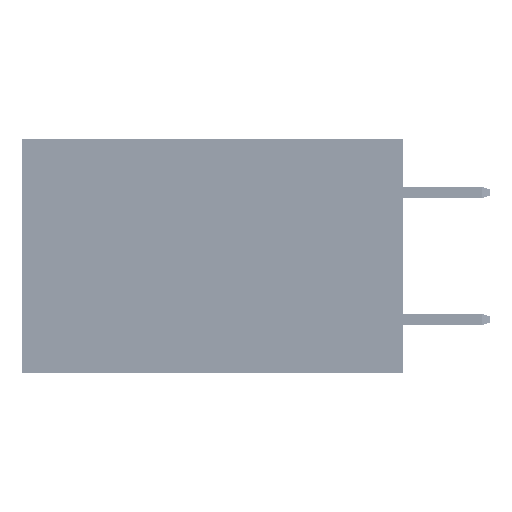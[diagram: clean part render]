
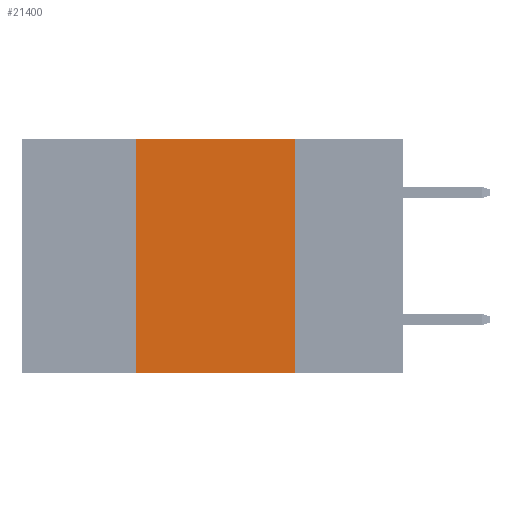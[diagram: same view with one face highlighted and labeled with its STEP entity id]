
A CAD part, left-side view. The second image highlights one B-rep face of the part: STEP entity #21400.
In plain terms, the highlighted planar face has unit normal (-1, 0, 0).
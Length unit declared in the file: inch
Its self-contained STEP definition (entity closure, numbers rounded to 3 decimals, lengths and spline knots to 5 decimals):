
#2221 = VERTEX_POINT ( 'NONE', #44517 ) ;
#2843 = CARTESIAN_POINT ( 'NONE',  ( 0., 0.17, 0. ) ) ;
#5233 = ORIENTED_EDGE ( 'NONE', *, *, #7562, .F. ) ;
#5838 = CARTESIAN_POINT ( 'NONE',  ( 0., 0.6, 0. ) ) ;
#6639 = CARTESIAN_POINT ( 'NONE',  ( 0., 0.6, -0.37 ) ) ;
#7511 = DIRECTION ( 'NONE',  ( 1., 0., 0. ) ) ;
#7562 = EDGE_CURVE ( 'NONE', #13985, #13422, #18154, .T. ) ;
#7747 = DIRECTION ( 'NONE',  ( 0., 0., -1. ) ) ;
#9118 = CARTESIAN_POINT ( 'NONE',  ( 0., 0.42, 0. ) ) ;
#10121 = EDGE_LOOP ( 'NONE', ( #5233, #22843, #23729, #23962 ) ) ;
#10524 = LINE ( 'NONE', #6639, #26430 ) ;
#12177 = EDGE_CURVE ( 'NONE', #27322, #13985, #42344, .T. ) ;
#12976 = VECTOR ( 'NONE', #14503, 39.37008 ) ;
#12993 = DIRECTION ( 'NONE',  ( 0., 0., 1. ) ) ;
#13153 = PLANE ( 'NONE',  #47562 ) ;
#13422 = VERTEX_POINT ( 'NONE', #26104 ) ;
#13985 = VERTEX_POINT ( 'NONE', #42999 ) ;
#14503 = DIRECTION ( 'NONE',  ( 0., 0., -1. ) ) ;
#17574 = DIRECTION ( 'NONE',  ( 0., -1., 0. ) ) ;
#18154 = LINE ( 'NONE', #2843, #12976 ) ;
#20473 = FACE_OUTER_BOUND ( 'NONE', #10121, .T. ) ;
#20960 = VECTOR ( 'NONE', #34807, 39.37008 ) ;
#21400 = ADVANCED_FACE ( 'NONE', ( #20473 ), #13153, .F. ) ;
#22475 = CARTESIAN_POINT ( 'NONE',  ( 0., 0.42, 0. ) ) ;
#22843 = ORIENTED_EDGE ( 'NONE', *, *, #12177, .F. ) ;
#23729 = ORIENTED_EDGE ( 'NONE', *, *, #27154, .F. ) ;
#23962 = ORIENTED_EDGE ( 'NONE', *, *, #46224, .T. ) ;
#26104 = CARTESIAN_POINT ( 'NONE',  ( 0., 0.17, -0.37 ) ) ;
#26430 = VECTOR ( 'NONE', #17574, 39.37008 ) ;
#27154 = EDGE_CURVE ( 'NONE', #2221, #27322, #27625, .T. ) ;
#27322 = VERTEX_POINT ( 'NONE', #22475 ) ;
#27625 = LINE ( 'NONE', #9118, #30029 ) ;
#30029 = VECTOR ( 'NONE', #12993, 39.37008 ) ;
#30143 = CARTESIAN_POINT ( 'NONE',  ( 0., 0.6, 0. ) ) ;
#34807 = DIRECTION ( 'NONE',  ( 0., -1., 0. ) ) ;
#42344 = LINE ( 'NONE', #5838, #20960 ) ;
#42999 = CARTESIAN_POINT ( 'NONE',  ( 0., 0.17, 0. ) ) ;
#44517 = CARTESIAN_POINT ( 'NONE',  ( 0., 0.42, -0.37 ) ) ;
#46224 = EDGE_CURVE ( 'NONE', #2221, #13422, #10524, .T. ) ;
#47562 = AXIS2_PLACEMENT_3D ( 'NONE', #30143, #7511, #7747 ) ;
